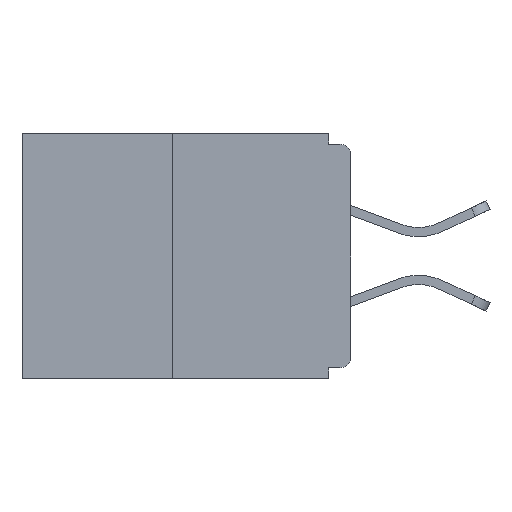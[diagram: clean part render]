
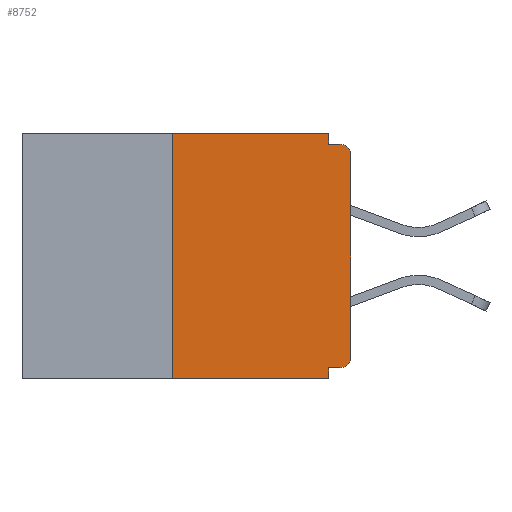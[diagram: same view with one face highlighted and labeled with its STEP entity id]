
A CAD part, left-side view. The second image highlights one B-rep face of the part: STEP entity #8752.
In plain terms, the highlighted planar face has unit normal (-1, 0, 0).
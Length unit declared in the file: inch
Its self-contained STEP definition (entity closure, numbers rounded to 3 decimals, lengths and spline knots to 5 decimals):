
#42 = ORIENTED_EDGE ( 'NONE', *, *, #8264, .F. ) ;
#176 = AXIS2_PLACEMENT_3D ( 'NONE', #23424, #7649, #11591 ) ;
#695 = EDGE_CURVE ( 'NONE', #19296, #10012, #23506, .T. ) ;
#712 = CARTESIAN_POINT ( 'NONE',  ( 0., 0.031, 0. ) ) ;
#944 = LINE ( 'NONE', #17184, #3671 ) ;
#1138 = CARTESIAN_POINT ( 'NONE',  ( 0., 0.031, -0.343 ) ) ;
#1325 = CARTESIAN_POINT ( 'NONE',  ( 0., 0., -0.313 ) ) ;
#1474 = VECTOR ( 'NONE', #12811, 39.37008 ) ;
#1654 = LINE ( 'NONE', #14829, #3803 ) ;
#1832 = VERTEX_POINT ( 'NONE', #1138 ) ;
#2052 = VERTEX_POINT ( 'NONE', #4473 ) ;
#2064 = VERTEX_POINT ( 'NONE', #712 ) ;
#2929 = DIRECTION ( 'NONE',  ( 0., 0., -1. ) ) ;
#3337 = EDGE_CURVE ( 'NONE', #5509, #1832, #17510, .T. ) ;
#3600 = EDGE_CURVE ( 'NONE', #10270, #1832, #25236, .T. ) ;
#3671 = VECTOR ( 'NONE', #5413, 39.37008 ) ;
#3704 = ORIENTED_EDGE ( 'NONE', *, *, #19085, .F. ) ;
#3803 = VECTOR ( 'NONE', #16874, 39.37008 ) ;
#3839 = VERTEX_POINT ( 'NONE', #1325 ) ;
#4473 = CARTESIAN_POINT ( 'NONE',  ( 0., 0.031, -0.015 ) ) ;
#5029 = ORIENTED_EDGE ( 'NONE', *, *, #19440, .F. ) ;
#5413 = DIRECTION ( 'NONE',  ( 0., 0., -1. ) ) ;
#5429 = LINE ( 'NONE', #21814, #19294 ) ;
#5509 = VERTEX_POINT ( 'NONE', #11656 ) ;
#6696 = DIRECTION ( 'NONE',  ( 1., 0., 0. ) ) ;
#7596 = LINE ( 'NONE', #14595, #13145 ) ;
#7649 = DIRECTION ( 'NONE',  ( -1., 0., 0. ) ) ;
#8264 = EDGE_CURVE ( 'NONE', #2052, #10012, #25272, .T. ) ;
#8579 = CARTESIAN_POINT ( 'NONE',  ( 0., 0.46, 0. ) ) ;
#8580 = DIRECTION ( 'NONE',  ( 0., 0., -1. ) ) ;
#8752 = ADVANCED_FACE ( 'NONE', ( #19651 ), #18719, .F. ) ;
#8961 = DIRECTION ( 'NONE',  ( -1., 0., 0. ) ) ;
#9803 = CARTESIAN_POINT ( 'NONE',  ( 0., 0.031, -0.328 ) ) ;
#10012 = VERTEX_POINT ( 'NONE', #16631 ) ;
#10239 = ORIENTED_EDGE ( 'NONE', *, *, #25076, .F. ) ;
#10270 = VERTEX_POINT ( 'NONE', #9803 ) ;
#10569 = CARTESIAN_POINT ( 'NONE',  ( 0., 0.46, -0.343 ) ) ;
#10599 = ORIENTED_EDGE ( 'NONE', *, *, #23057, .F. ) ;
#10619 = DIRECTION ( 'NONE',  ( 0., 0., 1. ) ) ;
#11591 = DIRECTION ( 'NONE',  ( 0., 0., -1. ) ) ;
#11656 = CARTESIAN_POINT ( 'NONE',  ( 0., 0.25, -0.343 ) ) ;
#12051 = ORIENTED_EDGE ( 'NONE', *, *, #13488, .T. ) ;
#12142 = CIRCLE ( 'NONE', #20169, 0.015 ) ;
#12534 = DIRECTION ( 'NONE',  ( 0., 0., -1. ) ) ;
#12811 = DIRECTION ( 'NONE',  ( 0., -1., 0. ) ) ;
#12857 = CARTESIAN_POINT ( 'NONE',  ( 0., 0., 0. ) ) ;
#13145 = VECTOR ( 'NONE', #14418, 39.37008 ) ;
#13216 = VECTOR ( 'NONE', #23901, 39.37008 ) ;
#13488 = EDGE_CURVE ( 'NONE', #3839, #19296, #17787, .T. ) ;
#13510 = CARTESIAN_POINT ( 'NONE',  ( 0., 0.25, 0. ) ) ;
#14418 = DIRECTION ( 'NONE',  ( 0., -1., 0. ) ) ;
#14595 = CARTESIAN_POINT ( 'NONE',  ( 0., 0.46, 0. ) ) ;
#14829 = CARTESIAN_POINT ( 'NONE',  ( 0., 0., -0.328 ) ) ;
#15572 = DIRECTION ( 'NONE',  ( 0., 0., 1. ) ) ;
#16253 = VECTOR ( 'NONE', #8580, 39.37008 ) ;
#16631 = CARTESIAN_POINT ( 'NONE',  ( 0., 0.015, -0.015 ) ) ;
#16874 = DIRECTION ( 'NONE',  ( 0., 1., 0. ) ) ;
#17062 = CARTESIAN_POINT ( 'NONE',  ( 0., 0., -0.03 ) ) ;
#17184 = CARTESIAN_POINT ( 'NONE',  ( 0., 0.031, 0. ) ) ;
#17510 = LINE ( 'NONE', #10569, #1474 ) ;
#17787 = LINE ( 'NONE', #12857, #18118 ) ;
#18118 = VECTOR ( 'NONE', #10619, 39.37008 ) ;
#18719 = PLANE ( 'NONE',  #22843 ) ;
#19085 = EDGE_CURVE ( 'NONE', #24392, #2064, #7596, .T. ) ;
#19144 = ORIENTED_EDGE ( 'NONE', *, *, #3337, .T. ) ;
#19294 = VECTOR ( 'NONE', #15572, 39.37008 ) ;
#19296 = VERTEX_POINT ( 'NONE', #17062 ) ;
#19440 = EDGE_CURVE ( 'NONE', #5509, #24392, #5429, .T. ) ;
#19651 = FACE_OUTER_BOUND ( 'NONE', #23470, .T. ) ;
#19659 = CARTESIAN_POINT ( 'NONE',  ( 0., 0.015, -0.328 ) ) ;
#19687 = ORIENTED_EDGE ( 'NONE', *, *, #25061, .T. ) ;
#20169 = AXIS2_PLACEMENT_3D ( 'NONE', #20538, #8961, #2929 ) ;
#20363 = CARTESIAN_POINT ( 'NONE',  ( 0., 0., -0.015 ) ) ;
#20399 = CARTESIAN_POINT ( 'NONE',  ( 0., 0.031, -0.343 ) ) ;
#20538 = CARTESIAN_POINT ( 'NONE',  ( 0., 0.015, -0.313 ) ) ;
#21524 = ORIENTED_EDGE ( 'NONE', *, *, #3600, .F. ) ;
#21814 = CARTESIAN_POINT ( 'NONE',  ( 0., 0.25, 0. ) ) ;
#22075 = ORIENTED_EDGE ( 'NONE', *, *, #695, .T. ) ;
#22843 = AXIS2_PLACEMENT_3D ( 'NONE', #8579, #6696, #12534 ) ;
#23057 = EDGE_CURVE ( 'NONE', #2064, #2052, #944, .T. ) ;
#23424 = CARTESIAN_POINT ( 'NONE',  ( 0., 0.015, -0.03 ) ) ;
#23470 = EDGE_LOOP ( 'NONE', ( #3704, #5029, #19144, #21524, #10239, #19687, #12051, #22075, #42, #10599 ) ) ;
#23506 = CIRCLE ( 'NONE', #176, 0.015 ) ;
#23901 = DIRECTION ( 'NONE',  ( 0., -1., 0. ) ) ;
#24009 = VERTEX_POINT ( 'NONE', #19659 ) ;
#24392 = VERTEX_POINT ( 'NONE', #13510 ) ;
#25061 = EDGE_CURVE ( 'NONE', #24009, #3839, #12142, .T. ) ;
#25076 = EDGE_CURVE ( 'NONE', #24009, #10270, #1654, .T. ) ;
#25236 = LINE ( 'NONE', #20399, #16253 ) ;
#25272 = LINE ( 'NONE', #20363, #13216 ) ;
